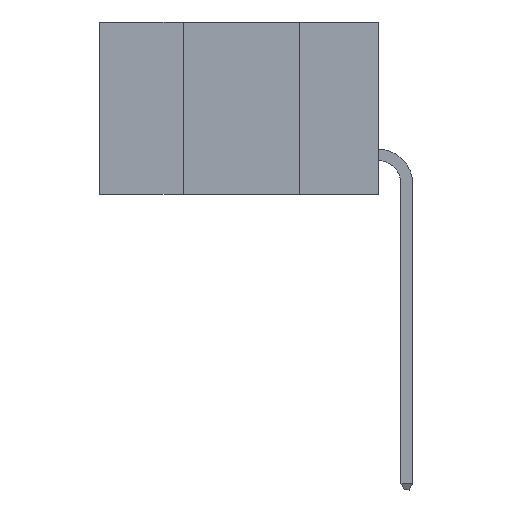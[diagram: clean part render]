
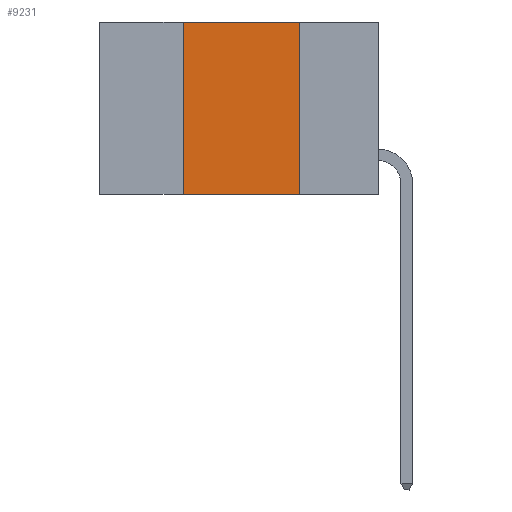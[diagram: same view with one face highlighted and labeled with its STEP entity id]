
A CAD part, left-side view. The second image highlights one B-rep face of the part: STEP entity #9231.
In plain terms, the highlighted planar face has unit normal (-1, 0, 0).
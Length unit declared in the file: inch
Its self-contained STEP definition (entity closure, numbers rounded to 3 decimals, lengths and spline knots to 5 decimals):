
#104 = VERTEX_POINT ( 'NONE', #2368 ) ;
#385 = CARTESIAN_POINT ( 'NONE',  ( 0., 0.17, 0. ) ) ;
#482 = ORIENTED_EDGE ( 'NONE', *, *, #3114, .F. ) ;
#2126 = EDGE_CURVE ( 'NONE', #104, #11343, #11633, .T. ) ;
#2368 = CARTESIAN_POINT ( 'NONE',  ( 0., 0.42, -0.37 ) ) ;
#2675 = DIRECTION ( 'NONE',  ( 0., 0., 1. ) ) ;
#2731 = DIRECTION ( 'NONE',  ( 0., -1., 0. ) ) ;
#2920 = VERTEX_POINT ( 'NONE', #6504 ) ;
#3114 = EDGE_CURVE ( 'NONE', #2920, #11343, #11980, .T. ) ;
#3206 = CARTESIAN_POINT ( 'NONE',  ( 0., 0.42, 0. ) ) ;
#4561 = VERTEX_POINT ( 'NONE', #3206 ) ;
#4569 = EDGE_LOOP ( 'NONE', ( #482, #4577, #10262, #6980 ) ) ;
#4577 = ORIENTED_EDGE ( 'NONE', *, *, #6790, .F. ) ;
#6504 = CARTESIAN_POINT ( 'NONE',  ( 0., 0.17, 0. ) ) ;
#6790 = EDGE_CURVE ( 'NONE', #4561, #2920, #14095, .T. ) ;
#6980 = ORIENTED_EDGE ( 'NONE', *, *, #2126, .T. ) ;
#7262 = FACE_OUTER_BOUND ( 'NONE', #4569, .T. ) ;
#8191 = CARTESIAN_POINT ( 'NONE',  ( 0., 0.42, 0. ) ) ;
#8202 = VECTOR ( 'NONE', #10698, 39.37008 ) ;
#8233 = DIRECTION ( 'NONE',  ( 0., 0., -1. ) ) ;
#8235 = DIRECTION ( 'NONE',  ( 1., 0., 0. ) ) ;
#8715 = VECTOR ( 'NONE', #2731, 39.37008 ) ;
#9052 = VECTOR ( 'NONE', #13161, 39.37008 ) ;
#9095 = VECTOR ( 'NONE', #2675, 39.37008 ) ;
#9231 = ADVANCED_FACE ( 'NONE', ( #7262 ), #12310, .F. ) ;
#9637 = CARTESIAN_POINT ( 'NONE',  ( 0., 0.17, -0.37 ) ) ;
#9786 = CARTESIAN_POINT ( 'NONE',  ( 0., 0.6, 0. ) ) ;
#10262 = ORIENTED_EDGE ( 'NONE', *, *, #11534, .F. ) ;
#10657 = AXIS2_PLACEMENT_3D ( 'NONE', #12299, #8235, #8233 ) ;
#10698 = DIRECTION ( 'NONE',  ( 0., -1., 0. ) ) ;
#10876 = CARTESIAN_POINT ( 'NONE',  ( 0., 0.6, -0.37 ) ) ;
#11343 = VERTEX_POINT ( 'NONE', #9637 ) ;
#11534 = EDGE_CURVE ( 'NONE', #104, #4561, #11660, .T. ) ;
#11633 = LINE ( 'NONE', #10876, #8715 ) ;
#11660 = LINE ( 'NONE', #8191, #9095 ) ;
#11980 = LINE ( 'NONE', #385, #9052 ) ;
#12299 = CARTESIAN_POINT ( 'NONE',  ( 0., 0.6, 0. ) ) ;
#12310 = PLANE ( 'NONE',  #10657 ) ;
#13161 = DIRECTION ( 'NONE',  ( 0., 0., -1. ) ) ;
#14095 = LINE ( 'NONE', #9786, #8202 ) ;
